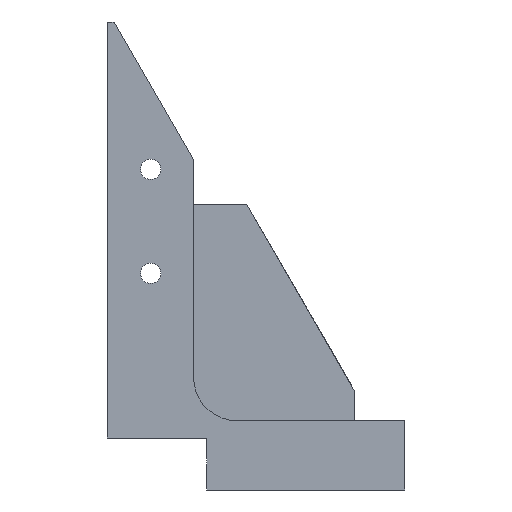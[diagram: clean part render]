
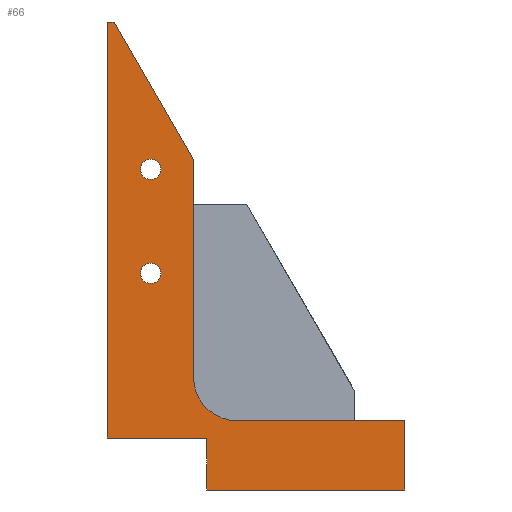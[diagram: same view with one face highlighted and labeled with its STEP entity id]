
A CAD part, left-side view. The second image highlights one B-rep face of the part: STEP entity #66.
In plain terms, the highlighted planar face has unit normal (-1, 0, 0).
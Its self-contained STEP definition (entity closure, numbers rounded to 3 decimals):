
#30 = ORIENTED_EDGE ( 'NONE', *, *, #892, .T. ) ;
#46 = CARTESIAN_POINT ( 'NONE',  ( -8.763, 30.931, 16.51 ) ) ;
#49 = DIRECTION ( 'NONE',  ( 0., 0., -1. ) ) ;
#56 = DIRECTION ( 'NONE',  ( 1., 0., 0. ) ) ;
#66 = ADVANCED_FACE ( 'NONE', ( #862, #89, #905 ), #821, .F. ) ;
#68 = VERTEX_POINT ( 'NONE', #805 ) ;
#73 = CARTESIAN_POINT ( 'NONE',  ( -8.763, 37.211, 31.75 ) ) ;
#78 = AXIS2_PLACEMENT_3D ( 'NONE', #73, #56, #49 ) ;
#87 = DIRECTION ( 'NONE',  ( 0., 0., -1. ) ) ;
#89 = FACE_BOUND ( 'NONE', #1054, .T. ) ;
#100 = CARTESIAN_POINT ( 'NONE',  ( -8.763, 37.211, 46.99 ) ) ;
#104 = DIRECTION ( 'NONE',  ( 1., 0., 0. ) ) ;
#115 = DIRECTION ( 'NONE',  ( 0., -1., 0. ) ) ;
#139 = VECTOR ( 'NONE', #1417, 1000. ) ;
#159 = LINE ( 'NONE', #672, #549 ) ;
#207 = VECTOR ( 'NONE', #929, 1000. ) ;
#209 = ORIENTED_EDGE ( 'NONE', *, *, #980, .T. ) ;
#289 = LINE ( 'NONE', #1668, #1010 ) ;
#318 = ORIENTED_EDGE ( 'NONE', *, *, #792, .T. ) ;
#382 = VECTOR ( 'NONE', #115, 1000. ) ;
#407 = EDGE_CURVE ( 'NONE', #1653, #1653, #1366, .T. ) ;
#426 = CARTESIAN_POINT ( 'NONE',  ( -8.763, 0., 10.16 ) ) ;
#429 = EDGE_CURVE ( 'NONE', #1325, #1325, #1291, .T. ) ;
#442 = CARTESIAN_POINT ( 'NONE',  ( -8.763, 29.026, 0. ) ) ;
#472 = CARTESIAN_POINT ( 'NONE',  ( -8.763, 37.211, 30.25 ) ) ;
#478 = LINE ( 'NONE', #1375, #1498 ) ;
#500 = EDGE_CURVE ( 'NONE', #1369, #1650, #1539, .T. ) ;
#504 = VERTEX_POINT ( 'NONE', #46 ) ;
#549 = VECTOR ( 'NONE', #665, 1000. ) ;
#595 = CARTESIAN_POINT ( 'NONE',  ( -8.763, 43.561, 7.62 ) ) ;
#626 = EDGE_CURVE ( 'NONE', #1650, #504, #1384, .T. ) ;
#639 = VERTEX_POINT ( 'NONE', #1155 ) ;
#665 = DIRECTION ( 'NONE',  ( 0., 0., -1. ) ) ;
#672 = CARTESIAN_POINT ( 'NONE',  ( -8.763, 29.026, 0. ) ) ;
#676 = ORIENTED_EDGE ( 'NONE', *, *, #429, .T. ) ;
#700 = EDGE_CURVE ( 'NONE', #504, #1166, #289, .T. ) ;
#701 = ORIENTED_EDGE ( 'NONE', *, *, #1550, .T. ) ;
#718 = ORIENTED_EDGE ( 'NONE', *, *, #626, .T. ) ;
#732 = LINE ( 'NONE', #1167, #1421 ) ;
#750 = CARTESIAN_POINT ( 'NONE',  ( -8.763, 0., 0. ) ) ;
#756 = CARTESIAN_POINT ( 'NONE',  ( -8.763, 0., 10.16 ) ) ;
#770 = LINE ( 'NONE', #1681, #382 ) ;
#792 = EDGE_CURVE ( 'NONE', #1166, #843, #906, .T. ) ;
#805 = CARTESIAN_POINT ( 'NONE',  ( -8.763, 43.561, 68.58 ) ) ;
#815 = EDGE_CURVE ( 'NONE', #843, #68, #478, .T. ) ;
#821 = PLANE ( 'NONE',  #1019 ) ;
#831 = DIRECTION ( 'NONE',  ( 0., 1., 0. ) ) ;
#840 = CARTESIAN_POINT ( 'NONE',  ( -8.763, 0., 0. ) ) ;
#843 = VERTEX_POINT ( 'NONE', #1378 ) ;
#844 = DIRECTION ( 'NONE',  ( 1., 0., 0. ) ) ;
#846 = DIRECTION ( 'NONE',  ( 0., 0., -1. ) ) ;
#862 = FACE_BOUND ( 'NONE', #1478, .T. ) ;
#866 = ORIENTED_EDGE ( 'NONE', *, *, #1038, .T. ) ;
#892 = EDGE_CURVE ( 'NONE', #68, #1059, #732, .T. ) ;
#905 = FACE_OUTER_BOUND ( 'NONE', #1627, .T. ) ;
#906 = LINE ( 'NONE', #1469, #139 ) ;
#920 = CARTESIAN_POINT ( 'NONE',  ( -8.763, 0., 7.62 ) ) ;
#929 = DIRECTION ( 'NONE',  ( 0., -1., 0. ) ) ;
#934 = CARTESIAN_POINT ( 'NONE',  ( -8.763, 0., 0. ) ) ;
#945 = DIRECTION ( 'NONE',  ( 0., 0., 1. ) ) ;
#960 = EDGE_CURVE ( 'NONE', #1029, #1369, #1014, .T. ) ;
#971 = VECTOR ( 'NONE', #945, 1000. ) ;
#980 = EDGE_CURVE ( 'NONE', #1059, #639, #1277, .T. ) ;
#1010 = VECTOR ( 'NONE', #1628, 1000. ) ;
#1014 = LINE ( 'NONE', #934, #971 ) ;
#1019 = AXIS2_PLACEMENT_3D ( 'NONE', #840, #844, #846 ) ;
#1029 = VERTEX_POINT ( 'NONE', #750 ) ;
#1038 = EDGE_CURVE ( 'NONE', #639, #1073, #159, .T. ) ;
#1045 = ORIENTED_EDGE ( 'NONE', *, *, #407, .T. ) ;
#1054 = EDGE_LOOP ( 'NONE', ( #676 ) ) ;
#1059 = VERTEX_POINT ( 'NONE', #595 ) ;
#1073 = VERTEX_POINT ( 'NONE', #442 ) ;
#1133 = CARTESIAN_POINT ( 'NONE',  ( -8.763, 24.581, 10.16 ) ) ;
#1142 = DIRECTION ( 'NONE',  ( 0., 0., -1. ) ) ;
#1155 = CARTESIAN_POINT ( 'NONE',  ( -8.763, 29.026, 7.62 ) ) ;
#1158 = DIRECTION ( 'NONE',  ( 0., 0., -1. ) ) ;
#1161 = CARTESIAN_POINT ( 'NONE',  ( -8.763, 30.931, 48.463 ) ) ;
#1163 = DIRECTION ( 'NONE',  ( 1., 0., 0. ) ) ;
#1166 = VERTEX_POINT ( 'NONE', #1161 ) ;
#1167 = CARTESIAN_POINT ( 'NONE',  ( -8.763, 43.561, 0. ) ) ;
#1190 = VECTOR ( 'NONE', #831, 1000. ) ;
#1196 = AXIS2_PLACEMENT_3D ( 'NONE', #1525, #1163, #1158 ) ;
#1197 = ORIENTED_EDGE ( 'NONE', *, *, #960, .T. ) ;
#1263 = CARTESIAN_POINT ( 'NONE',  ( -8.763, 37.211, 45.49 ) ) ;
#1277 = LINE ( 'NONE', #920, #207 ) ;
#1291 = CIRCLE ( 'NONE', #78, 1.5 ) ;
#1325 = VERTEX_POINT ( 'NONE', #472 ) ;
#1366 = CIRCLE ( 'NONE', #1699, 1.5 ) ;
#1369 = VERTEX_POINT ( 'NONE', #426 ) ;
#1375 = CARTESIAN_POINT ( 'NONE',  ( -8.763, 0., 68.58 ) ) ;
#1378 = CARTESIAN_POINT ( 'NONE',  ( -8.763, 42.545, 68.58 ) ) ;
#1384 = CIRCLE ( 'NONE', #1196, 6.35 ) ;
#1386 = DIRECTION ( 'NONE',  ( 0., 1., 0. ) ) ;
#1417 = DIRECTION ( 'NONE',  ( 0., 0.5, 0.866 ) ) ;
#1421 = VECTOR ( 'NONE', #1142, 1000. ) ;
#1424 = ORIENTED_EDGE ( 'NONE', *, *, #500, .T. ) ;
#1469 = CARTESIAN_POINT ( 'NONE',  ( -8.763, 2.213, -1.278 ) ) ;
#1478 = EDGE_LOOP ( 'NONE', ( #1045 ) ) ;
#1498 = VECTOR ( 'NONE', #1386, 1000. ) ;
#1508 = ORIENTED_EDGE ( 'NONE', *, *, #700, .T. ) ;
#1525 = CARTESIAN_POINT ( 'NONE',  ( -8.763, 24.581, 16.51 ) ) ;
#1539 = LINE ( 'NONE', #756, #1190 ) ;
#1550 = EDGE_CURVE ( 'NONE', #1073, #1029, #770, .T. ) ;
#1585 = ORIENTED_EDGE ( 'NONE', *, *, #815, .T. ) ;
#1627 = EDGE_LOOP ( 'NONE', ( #1424, #718, #1508, #318, #1585, #30, #209, #866, #701, #1197 ) ) ;
#1628 = DIRECTION ( 'NONE',  ( 0., 0., 1. ) ) ;
#1650 = VERTEX_POINT ( 'NONE', #1133 ) ;
#1653 = VERTEX_POINT ( 'NONE', #1263 ) ;
#1668 = CARTESIAN_POINT ( 'NONE',  ( -8.763, 30.931, 0. ) ) ;
#1681 = CARTESIAN_POINT ( 'NONE',  ( -8.763, 0., 0. ) ) ;
#1699 = AXIS2_PLACEMENT_3D ( 'NONE', #100, #104, #87 ) ;
